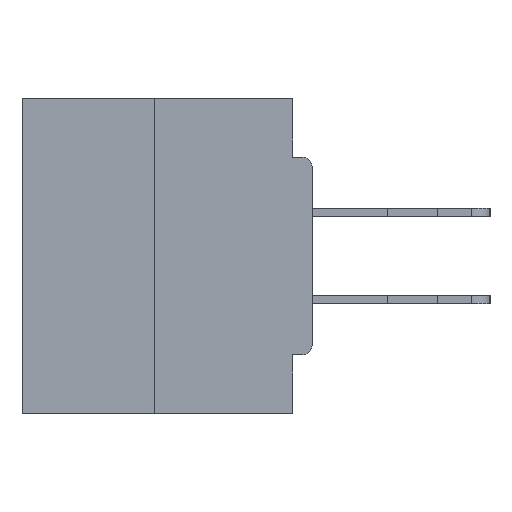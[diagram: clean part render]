
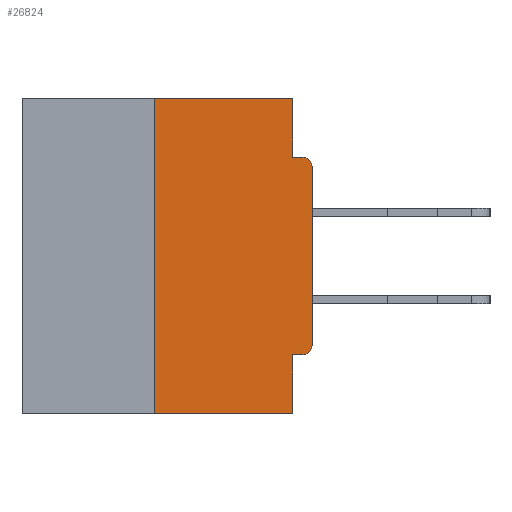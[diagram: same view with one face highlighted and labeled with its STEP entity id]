
A CAD part, left-side view. The second image highlights one B-rep face of the part: STEP entity #26824.
In plain terms, the highlighted planar face has unit normal (-1, 0, 0).
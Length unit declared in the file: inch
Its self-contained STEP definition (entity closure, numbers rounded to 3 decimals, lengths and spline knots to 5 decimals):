
#18 = VERTEX_POINT ( 'NONE', #12663 ) ;
#80 = VECTOR ( 'NONE', #15759, 39.37008 ) ;
#239 = DIRECTION ( 'NONE',  ( 0., 0., -1. ) ) ;
#462 = VERTEX_POINT ( 'NONE', #5451 ) ;
#821 = VECTOR ( 'NONE', #19149, 39.37008 ) ;
#1340 = VERTEX_POINT ( 'NONE', #33865 ) ;
#2884 = DIRECTION ( 'NONE',  ( 0., 0., 1. ) ) ;
#3204 = CIRCLE ( 'NONE', #23183, 0.015 ) ;
#4795 = CARTESIAN_POINT ( 'NONE',  ( 0., 0.46, -0.5 ) ) ;
#4936 = EDGE_CURVE ( 'NONE', #12503, #9266, #18248, .T. ) ;
#5451 = CARTESIAN_POINT ( 'NONE',  ( 0., 0.25, 0. ) ) ;
#6588 = FACE_OUTER_BOUND ( 'NONE', #22532, .T. ) ;
#7101 = ORIENTED_EDGE ( 'NONE', *, *, #4936, .F. ) ;
#7448 = CARTESIAN_POINT ( 'NONE',  ( 0., 0.031, -0.5 ) ) ;
#7461 = LINE ( 'NONE', #4795, #15176 ) ;
#8368 = ORIENTED_EDGE ( 'NONE', *, *, #32765, .T. ) ;
#8503 = DIRECTION ( 'NONE',  ( 0., 0., -1. ) ) ;
#9266 = VERTEX_POINT ( 'NONE', #25453 ) ;
#9828 = EDGE_CURVE ( 'NONE', #15314, #18, #31513, .T. ) ;
#10556 = LINE ( 'NONE', #21495, #80 ) ;
#10698 = CARTESIAN_POINT ( 'NONE',  ( 0., 0.25, -0.5 ) ) ;
#11561 = PLANE ( 'NONE',  #25382 ) ;
#11585 = ORIENTED_EDGE ( 'NONE', *, *, #14088, .F. ) ;
#12067 = VECTOR ( 'NONE', #20941, 39.37008 ) ;
#12093 = CARTESIAN_POINT ( 'NONE',  ( 0., 0.46, 0. ) ) ;
#12503 = VERTEX_POINT ( 'NONE', #24227 ) ;
#12663 = CARTESIAN_POINT ( 'NONE',  ( 0., 0.031, -0.4065 ) ) ;
#12870 = CARTESIAN_POINT ( 'NONE',  ( 0., 0., -0.4065 ) ) ;
#13207 = CARTESIAN_POINT ( 'NONE',  ( 0., 0., 0. ) ) ;
#13304 = VERTEX_POINT ( 'NONE', #35014 ) ;
#14088 = EDGE_CURVE ( 'NONE', #26782, #462, #16454, .T. ) ;
#14133 = EDGE_CURVE ( 'NONE', #462, #20157, #10556, .T. ) ;
#14620 = DIRECTION ( 'NONE',  ( 1., 0., 0. ) ) ;
#15176 = VECTOR ( 'NONE', #15861, 39.37008 ) ;
#15314 = VERTEX_POINT ( 'NONE', #24591 ) ;
#15470 = VECTOR ( 'NONE', #2884, 39.37008 ) ;
#15759 = DIRECTION ( 'NONE',  ( 0., -1., 0. ) ) ;
#15861 = DIRECTION ( 'NONE',  ( 0., -1., 0. ) ) ;
#15921 = ORIENTED_EDGE ( 'NONE', *, *, #9828, .F. ) ;
#16454 = LINE ( 'NONE', #32594, #15470 ) ;
#17332 = CIRCLE ( 'NONE', #28778, 0.015 ) ;
#18248 = LINE ( 'NONE', #23957, #12067 ) ;
#18459 = CARTESIAN_POINT ( 'NONE',  ( 0., 0.031, 0. ) ) ;
#19149 = DIRECTION ( 'NONE',  ( 0., 0., 1. ) ) ;
#19299 = EDGE_CURVE ( 'NONE', #18, #33804, #26408, .T. ) ;
#19398 = DIRECTION ( 'NONE',  ( 0., 0., -1. ) ) ;
#19710 = CARTESIAN_POINT ( 'NONE',  ( 0., 0.031, 0. ) ) ;
#20157 = VERTEX_POINT ( 'NONE', #18459 ) ;
#20701 = DIRECTION ( 'NONE',  ( 0., 0., -1. ) ) ;
#20941 = DIRECTION ( 'NONE',  ( 0., -1., 0. ) ) ;
#21495 = CARTESIAN_POINT ( 'NONE',  ( 0., 0.46, 0. ) ) ;
#22090 = ORIENTED_EDGE ( 'NONE', *, *, #33251, .T. ) ;
#22119 = CARTESIAN_POINT ( 'NONE',  ( 0., 0.015, -0.1085 ) ) ;
#22263 = DIRECTION ( 'NONE',  ( -1., 0., 0. ) ) ;
#22319 = VECTOR ( 'NONE', #34385, 39.37008 ) ;
#22532 = EDGE_LOOP ( 'NONE', ( #26447, #11585, #30774, #31079, #15921, #8368, #22090, #25903, #7101, #27793 ) ) ;
#22569 = LINE ( 'NONE', #19710, #27529 ) ;
#23183 = AXIS2_PLACEMENT_3D ( 'NONE', #22119, #33049, #8503 ) ;
#23957 = CARTESIAN_POINT ( 'NONE',  ( 0., 0., -0.0935 ) ) ;
#24227 = CARTESIAN_POINT ( 'NONE',  ( 0., 0.031, -0.0935 ) ) ;
#24591 = CARTESIAN_POINT ( 'NONE',  ( 0., 0.015, -0.4065 ) ) ;
#25382 = AXIS2_PLACEMENT_3D ( 'NONE', #12093, #14620, #33448 ) ;
#25453 = CARTESIAN_POINT ( 'NONE',  ( 0., 0.015, -0.0935 ) ) ;
#25903 = ORIENTED_EDGE ( 'NONE', *, *, #28497, .T. ) ;
#26408 = LINE ( 'NONE', #7448, #26846 ) ;
#26447 = ORIENTED_EDGE ( 'NONE', *, *, #14133, .F. ) ;
#26782 = VERTEX_POINT ( 'NONE', #10698 ) ;
#26824 = ADVANCED_FACE ( 'NONE', ( #6588 ), #11561, .F. ) ;
#26846 = VECTOR ( 'NONE', #20701, 39.37008 ) ;
#27529 = VECTOR ( 'NONE', #239, 39.37008 ) ;
#27793 = ORIENTED_EDGE ( 'NONE', *, *, #30132, .F. ) ;
#28209 = CARTESIAN_POINT ( 'NONE',  ( 0., 0.031, -0.5 ) ) ;
#28383 = EDGE_CURVE ( 'NONE', #26782, #33804, #7461, .T. ) ;
#28497 = EDGE_CURVE ( 'NONE', #13304, #9266, #3204, .T. ) ;
#28778 = AXIS2_PLACEMENT_3D ( 'NONE', #33197, #22263, #19398 ) ;
#30132 = EDGE_CURVE ( 'NONE', #20157, #12503, #22569, .T. ) ;
#30774 = ORIENTED_EDGE ( 'NONE', *, *, #28383, .T. ) ;
#31079 = ORIENTED_EDGE ( 'NONE', *, *, #19299, .F. ) ;
#31513 = LINE ( 'NONE', #12870, #22319 ) ;
#32594 = CARTESIAN_POINT ( 'NONE',  ( 0., 0.25, 0. ) ) ;
#32765 = EDGE_CURVE ( 'NONE', #15314, #1340, #17332, .T. ) ;
#32941 = LINE ( 'NONE', #13207, #821 ) ;
#33049 = DIRECTION ( 'NONE',  ( -1., 0., 0. ) ) ;
#33197 = CARTESIAN_POINT ( 'NONE',  ( 0., 0.015, -0.3915 ) ) ;
#33251 = EDGE_CURVE ( 'NONE', #1340, #13304, #32941, .T. ) ;
#33448 = DIRECTION ( 'NONE',  ( 0., 0., -1. ) ) ;
#33804 = VERTEX_POINT ( 'NONE', #28209 ) ;
#33865 = CARTESIAN_POINT ( 'NONE',  ( 0., 0., -0.3915 ) ) ;
#34385 = DIRECTION ( 'NONE',  ( 0., 1., 0. ) ) ;
#35014 = CARTESIAN_POINT ( 'NONE',  ( 0., 0., -0.1085 ) ) ;
